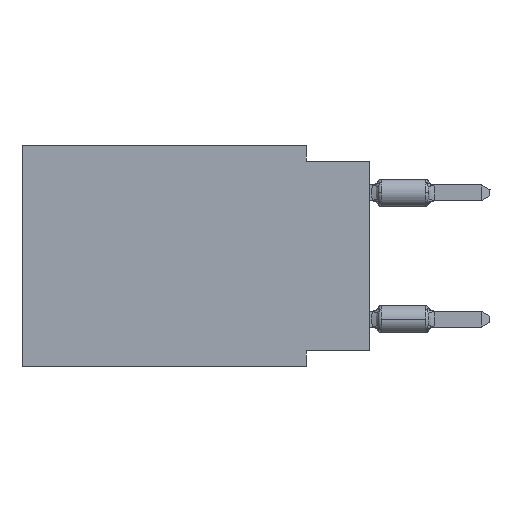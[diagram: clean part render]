
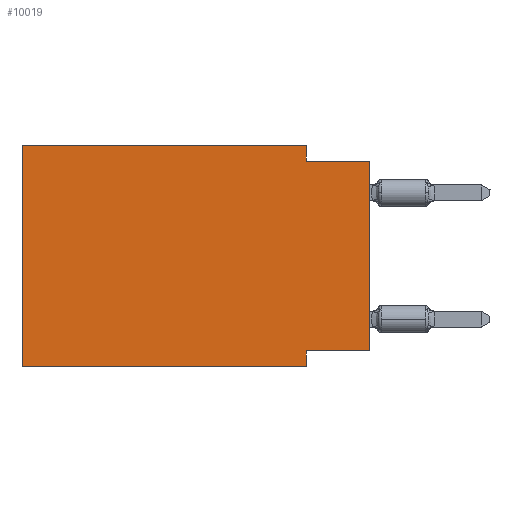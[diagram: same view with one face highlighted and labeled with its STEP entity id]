
A CAD part, left-side view. The second image highlights one B-rep face of the part: STEP entity #10019.
In plain terms, the highlighted planar face has unit normal (-1, 0, 0).
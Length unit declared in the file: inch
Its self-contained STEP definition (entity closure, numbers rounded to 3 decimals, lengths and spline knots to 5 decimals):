
#555 = CARTESIAN_POINT ( 'NONE',  ( 0., 0.55, 0. ) ) ;
#1072 = LINE ( 'NONE', #20098, #24870 ) ;
#1520 = VECTOR ( 'NONE', #8215, 39.37008 ) ;
#2447 = CARTESIAN_POINT ( 'NONE',  ( 0., 0.1, -0.35 ) ) ;
#2736 = VECTOR ( 'NONE', #33188, 39.37008 ) ;
#2745 = ORIENTED_EDGE ( 'NONE', *, *, #8556, .F. ) ;
#2923 = PLANE ( 'NONE',  #24028 ) ;
#3116 = DIRECTION ( 'NONE',  ( 0., 1., 0. ) ) ;
#3323 = DIRECTION ( 'NONE',  ( 0., 0., -1. ) ) ;
#3439 = LINE ( 'NONE', #6108, #25359 ) ;
#5585 = VERTEX_POINT ( 'NONE', #26331 ) ;
#5625 = VERTEX_POINT ( 'NONE', #5869 ) ;
#5777 = LINE ( 'NONE', #27464, #25433 ) ;
#5835 = CARTESIAN_POINT ( 'NONE',  ( 0., 0., -0.025 ) ) ;
#5869 = CARTESIAN_POINT ( 'NONE',  ( 0., 0., -0.325 ) ) ;
#5996 = LINE ( 'NONE', #27672, #29693 ) ;
#6108 = CARTESIAN_POINT ( 'NONE',  ( 0., 0.55, -0.35 ) ) ;
#6325 = VERTEX_POINT ( 'NONE', #22364 ) ;
#6607 = CARTESIAN_POINT ( 'NONE',  ( 0., 0.55, 0. ) ) ;
#7421 = VERTEX_POINT ( 'NONE', #5835 ) ;
#8215 = DIRECTION ( 'NONE',  ( 0., 0., 1. ) ) ;
#8540 = VERTEX_POINT ( 'NONE', #28655 ) ;
#8556 = EDGE_CURVE ( 'NONE', #6325, #9452, #18168, .T. ) ;
#8817 = EDGE_CURVE ( 'NONE', #5585, #32036, #1072, .T. ) ;
#8946 = EDGE_LOOP ( 'NONE', ( #24895, #11277, #17099, #10718, #9285, #31690, #2745, #16733 ) ) ;
#9285 = ORIENTED_EDGE ( 'NONE', *, *, #14194, .F. ) ;
#9452 = VERTEX_POINT ( 'NONE', #2447 ) ;
#9680 = EDGE_CURVE ( 'NONE', #32036, #31065, #5996, .T. ) ;
#10019 = ADVANCED_FACE ( 'NONE', ( #14773 ), #2923, .F. ) ;
#10516 = CARTESIAN_POINT ( 'NONE',  ( 0., 0., 0. ) ) ;
#10718 = ORIENTED_EDGE ( 'NONE', *, *, #8817, .F. ) ;
#11277 = ORIENTED_EDGE ( 'NONE', *, *, #26762, .F. ) ;
#11327 = LINE ( 'NONE', #30166, #2736 ) ;
#11394 = LINE ( 'NONE', #555, #1520 ) ;
#13808 = EDGE_CURVE ( 'NONE', #8540, #9452, #3439, .T. ) ;
#13946 = DIRECTION ( 'NONE',  ( 1., 0., 0. ) ) ;
#14194 = EDGE_CURVE ( 'NONE', #8540, #5585, #11394, .T. ) ;
#14773 = FACE_OUTER_BOUND ( 'NONE', #8946, .T. ) ;
#16000 = VECTOR ( 'NONE', #28997, 39.37008 ) ;
#16733 = ORIENTED_EDGE ( 'NONE', *, *, #27122, .F. ) ;
#17099 = ORIENTED_EDGE ( 'NONE', *, *, #9680, .F. ) ;
#18168 = LINE ( 'NONE', #31674, #16000 ) ;
#19895 = VECTOR ( 'NONE', #27213, 39.37008 ) ;
#20098 = CARTESIAN_POINT ( 'NONE',  ( 0., 0.55, 0. ) ) ;
#22364 = CARTESIAN_POINT ( 'NONE',  ( 0., 0.1, -0.325 ) ) ;
#22639 = DIRECTION ( 'NONE',  ( 0., -1., 0. ) ) ;
#24028 = AXIS2_PLACEMENT_3D ( 'NONE', #6607, #13946, #33790 ) ;
#24466 = CARTESIAN_POINT ( 'NONE',  ( 0., 0.1, 0. ) ) ;
#24870 = VECTOR ( 'NONE', #30412, 39.37008 ) ;
#24895 = ORIENTED_EDGE ( 'NONE', *, *, #29840, .T. ) ;
#25359 = VECTOR ( 'NONE', #22639, 39.37008 ) ;
#25433 = VECTOR ( 'NONE', #3116, 39.37008 ) ;
#26040 = CARTESIAN_POINT ( 'NONE',  ( 0., 0.1, -0.025 ) ) ;
#26331 = CARTESIAN_POINT ( 'NONE',  ( 0., 0.55, 0. ) ) ;
#26762 = EDGE_CURVE ( 'NONE', #31065, #7421, #11327, .T. ) ;
#27122 = EDGE_CURVE ( 'NONE', #5625, #6325, #5777, .T. ) ;
#27213 = DIRECTION ( 'NONE',  ( 0., 0., 1. ) ) ;
#27464 = CARTESIAN_POINT ( 'NONE',  ( 0., 0., -0.325 ) ) ;
#27672 = CARTESIAN_POINT ( 'NONE',  ( 0., 0.1, 0. ) ) ;
#28655 = CARTESIAN_POINT ( 'NONE',  ( 0., 0.55, -0.35 ) ) ;
#28997 = DIRECTION ( 'NONE',  ( 0., 0., -1. ) ) ;
#29341 = LINE ( 'NONE', #10516, #19895 ) ;
#29693 = VECTOR ( 'NONE', #3323, 39.37008 ) ;
#29840 = EDGE_CURVE ( 'NONE', #5625, #7421, #29341, .T. ) ;
#30166 = CARTESIAN_POINT ( 'NONE',  ( 0., 0., -0.025 ) ) ;
#30412 = DIRECTION ( 'NONE',  ( 0., -1., 0. ) ) ;
#31065 = VERTEX_POINT ( 'NONE', #26040 ) ;
#31674 = CARTESIAN_POINT ( 'NONE',  ( 0., 0.1, -0.35 ) ) ;
#31690 = ORIENTED_EDGE ( 'NONE', *, *, #13808, .T. ) ;
#32036 = VERTEX_POINT ( 'NONE', #24466 ) ;
#33188 = DIRECTION ( 'NONE',  ( 0., -1., 0. ) ) ;
#33790 = DIRECTION ( 'NONE',  ( 0., 0., -1. ) ) ;
